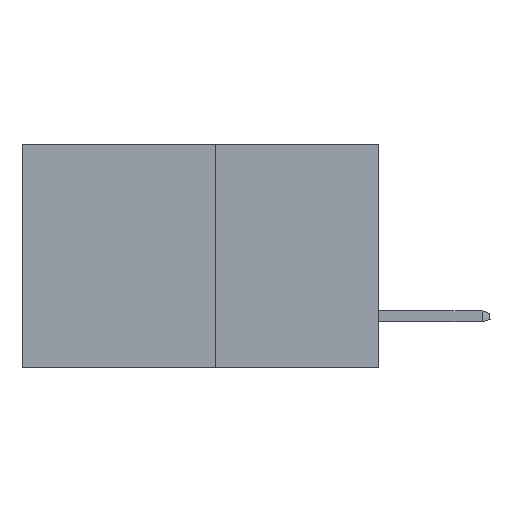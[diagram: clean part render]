
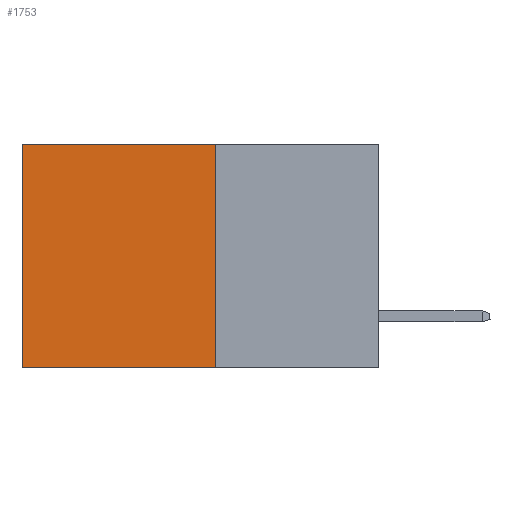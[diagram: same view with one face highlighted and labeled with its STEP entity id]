
A CAD part, left-side view. The second image highlights one B-rep face of the part: STEP entity #1753.
In plain terms, the highlighted planar face has unit normal (-1, 0, 0).
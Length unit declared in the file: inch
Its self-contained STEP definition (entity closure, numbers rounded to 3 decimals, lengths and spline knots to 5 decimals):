
#12 = ORIENTED_EDGE ( 'NONE', *, *, #16345, .F. ) ;
#371 = AXIS2_PLACEMENT_3D ( 'NONE', #5466, #20614, #20519 ) ;
#493 = CARTESIAN_POINT ( 'NONE',  ( 0.277, 0.59, -0.37 ) ) ;
#1295 = VECTOR ( 'NONE', #8198, 39.37008 ) ;
#1753 = ADVANCED_FACE ( 'NONE', ( #19401 ), #2667, .F. ) ;
#2667 = PLANE ( 'NONE',  #371 ) ;
#2715 = ORIENTED_EDGE ( 'NONE', *, *, #13480, .F. ) ;
#5105 = VERTEX_POINT ( 'NONE', #17336 ) ;
#5378 = CARTESIAN_POINT ( 'NONE',  ( 0.277, 0.27, 0. ) ) ;
#5466 = CARTESIAN_POINT ( 'NONE',  ( 0.277, 0.27, -0.37 ) ) ;
#6193 = LINE ( 'NONE', #9072, #19152 ) ;
#6706 = VERTEX_POINT ( 'NONE', #7462 ) ;
#7462 = CARTESIAN_POINT ( 'NONE',  ( 0.277, 0.27, 0. ) ) ;
#8198 = DIRECTION ( 'NONE',  ( 0., 0., -1. ) ) ;
#9072 = CARTESIAN_POINT ( 'NONE',  ( 0.277, 0.59, -0.37 ) ) ;
#9460 = ORIENTED_EDGE ( 'NONE', *, *, #15867, .T. ) ;
#10070 = EDGE_CURVE ( 'NONE', #5105, #11080, #6193, .T. ) ;
#11080 = VERTEX_POINT ( 'NONE', #493 ) ;
#11671 = LINE ( 'NONE', #17548, #14971 ) ;
#12749 = LINE ( 'NONE', #13111, #1295 ) ;
#13111 = CARTESIAN_POINT ( 'NONE',  ( 0.277, 0.27, -0.37 ) ) ;
#13480 = EDGE_CURVE ( 'NONE', #15119, #11080, #11671, .T. ) ;
#13784 = LINE ( 'NONE', #5378, #18110 ) ;
#14971 = VECTOR ( 'NONE', #19168, 39.37008 ) ;
#15119 = VERTEX_POINT ( 'NONE', #19741 ) ;
#15614 = DIRECTION ( 'NONE',  ( 0., 0., -1. ) ) ;
#15867 = EDGE_CURVE ( 'NONE', #6706, #5105, #13784, .T. ) ;
#16345 = EDGE_CURVE ( 'NONE', #6706, #15119, #12749, .T. ) ;
#17336 = CARTESIAN_POINT ( 'NONE',  ( 0.277, 0.59, 0. ) ) ;
#17548 = CARTESIAN_POINT ( 'NONE',  ( 0.277, 0.27, -0.37 ) ) ;
#17800 = ORIENTED_EDGE ( 'NONE', *, *, #10070, .T. ) ;
#18110 = VECTOR ( 'NONE', #18385, 39.37008 ) ;
#18385 = DIRECTION ( 'NONE',  ( 0., 1., 0. ) ) ;
#19152 = VECTOR ( 'NONE', #15614, 39.37008 ) ;
#19168 = DIRECTION ( 'NONE',  ( 0., 1., 0. ) ) ;
#19401 = FACE_OUTER_BOUND ( 'NONE', #19664, .T. ) ;
#19664 = EDGE_LOOP ( 'NONE', ( #17800, #2715, #12, #9460 ) ) ;
#19741 = CARTESIAN_POINT ( 'NONE',  ( 0.277, 0.27, -0.37 ) ) ;
#20519 = DIRECTION ( 'NONE',  ( 0., 0., -1. ) ) ;
#20614 = DIRECTION ( 'NONE',  ( 1., 0., 0. ) ) ;
